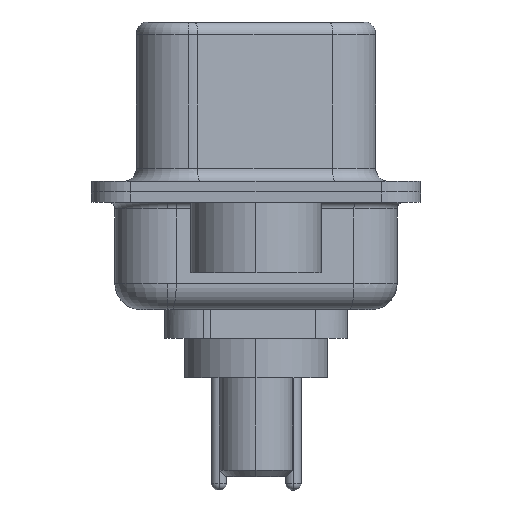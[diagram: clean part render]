
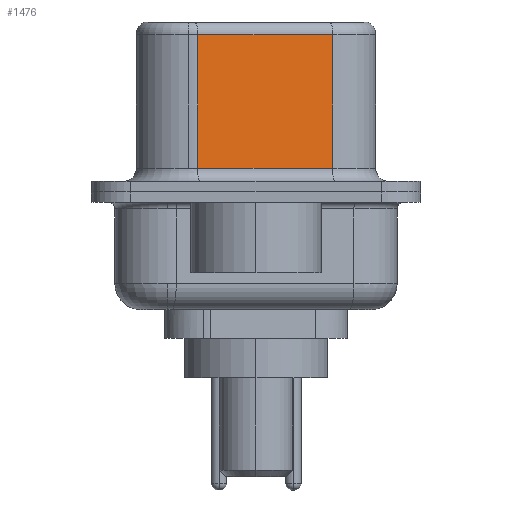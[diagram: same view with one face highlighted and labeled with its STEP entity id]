
A CAD part, left-side view. The second image highlights one B-rep face of the part: STEP entity #1476.
In plain terms, the highlighted planar face has unit normal (-0.985, -0.174, 0).
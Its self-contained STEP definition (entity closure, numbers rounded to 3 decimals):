
#294 = LINE ( 'NONE', #12643, #8962 ) ;
#696 = CARTESIAN_POINT ( 'NONE',  ( 4.585, -2.927, 0.9 ) ) ;
#1004 = DIRECTION ( 'NONE',  ( 0., 0., -1. ) ) ;
#1028 = EDGE_CURVE ( 'NONE', #5506, #4534, #294, .T. ) ;
#1476 = ADVANCED_FACE ( 'NONE', ( #1807 ), #11269, .F. ) ;
#1807 = FACE_OUTER_BOUND ( 'NONE', #8487, .T. ) ;
#1904 = CARTESIAN_POINT ( 'NONE',  ( 3.675, 2.233, 0.9 ) ) ;
#1988 = DIRECTION ( 'NONE',  ( 0., 0., -1. ) ) ;
#2097 = DIRECTION ( 'NONE',  ( 0.985, 0.174, 0. ) ) ;
#2342 = EDGE_CURVE ( 'NONE', #19585, #5506, #7401, .T. ) ;
#2872 = ORIENTED_EDGE ( 'NONE', *, *, #4641, .T. ) ;
#3013 = VECTOR ( 'NONE', #16509, 1000. ) ;
#4534 = VERTEX_POINT ( 'NONE', #1904 ) ;
#4641 = EDGE_CURVE ( 'NONE', #4534, #13949, #12121, .T. ) ;
#5506 = VERTEX_POINT ( 'NONE', #12633 ) ;
#5708 = ORIENTED_EDGE ( 'NONE', *, *, #1028, .T. ) ;
#6002 = CARTESIAN_POINT ( 'NONE',  ( 4.585, -2.927, 0.9 ) ) ;
#6888 = CARTESIAN_POINT ( 'NONE',  ( 4.585, -2.927, 6.52 ) ) ;
#7219 = EDGE_CURVE ( 'NONE', #19585, #13949, #19493, .T. ) ;
#7401 = LINE ( 'NONE', #11821, #19314 ) ;
#8100 = CARTESIAN_POINT ( 'NONE',  ( 4.585, -2.927, 6.02 ) ) ;
#8487 = EDGE_LOOP ( 'NONE', ( #19151, #16525, #5708, #2872 ) ) ;
#8962 = VECTOR ( 'NONE', #1004, 1000. ) ;
#10411 = DIRECTION ( 'NONE',  ( -0.174, 0.985, 0. ) ) ;
#11269 = PLANE ( 'NONE',  #16799 ) ;
#11821 = CARTESIAN_POINT ( 'NONE',  ( 4.585, -2.927, 6.02 ) ) ;
#12121 = LINE ( 'NONE', #696, #3013 ) ;
#12633 = CARTESIAN_POINT ( 'NONE',  ( 3.675, 2.233, 6.02 ) ) ;
#12643 = CARTESIAN_POINT ( 'NONE',  ( 3.675, 2.233, 6.52 ) ) ;
#13949 = VERTEX_POINT ( 'NONE', #6002 ) ;
#14157 = VECTOR ( 'NONE', #1988, 1000. ) ;
#16509 = DIRECTION ( 'NONE',  ( 0.174, -0.985, 0. ) ) ;
#16525 = ORIENTED_EDGE ( 'NONE', *, *, #2342, .T. ) ;
#16799 = AXIS2_PLACEMENT_3D ( 'NONE', #6888, #2097, #20519 ) ;
#18179 = CARTESIAN_POINT ( 'NONE',  ( 4.585, -2.927, 6.52 ) ) ;
#19151 = ORIENTED_EDGE ( 'NONE', *, *, #7219, .F. ) ;
#19314 = VECTOR ( 'NONE', #10411, 1000. ) ;
#19493 = LINE ( 'NONE', #18179, #14157 ) ;
#19585 = VERTEX_POINT ( 'NONE', #8100 ) ;
#20519 = DIRECTION ( 'NONE',  ( -0.174, 0.985, 0. ) ) ;
